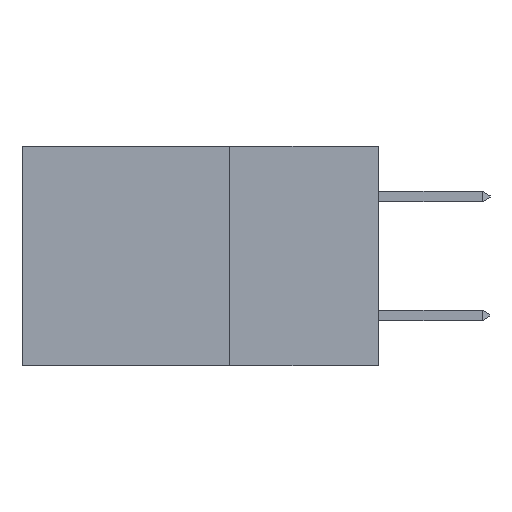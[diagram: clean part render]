
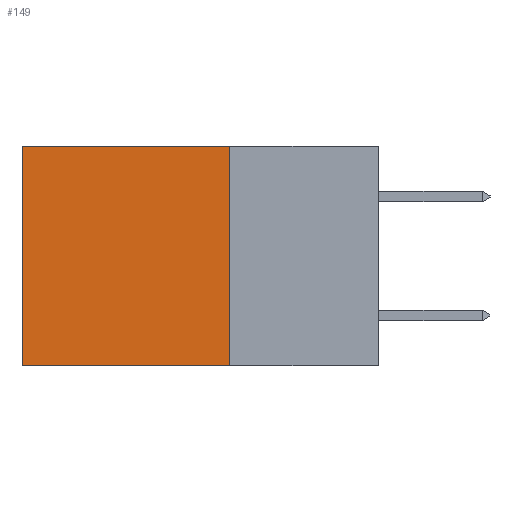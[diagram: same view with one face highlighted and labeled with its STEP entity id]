
A CAD part, left-side view. The second image highlights one B-rep face of the part: STEP entity #149.
In plain terms, the highlighted planar face has unit normal (-1, 0, 0).
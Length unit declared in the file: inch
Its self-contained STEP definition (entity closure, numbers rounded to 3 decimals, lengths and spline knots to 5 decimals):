
#149 = ADVANCED_FACE ( 'NONE', ( #1128 ), #3359, .F. ) ;
#1128 = FACE_OUTER_BOUND ( 'NONE', #11499, .T. ) ;
#1230 = CARTESIAN_POINT ( 'NONE',  ( 0.2615, 0.25, -0.37 ) ) ;
#1294 = DIRECTION ( 'NONE',  ( 0., 0., -1. ) ) ;
#1419 = DIRECTION ( 'NONE',  ( 0., 1., 0. ) ) ;
#2017 = CARTESIAN_POINT ( 'NONE',  ( 0.2615, 0.25, 0. ) ) ;
#2032 = LINE ( 'NONE', #10376, #15685 ) ;
#3327 = DIRECTION ( 'NONE',  ( 1., 0., 0. ) ) ;
#3359 = PLANE ( 'NONE',  #15931 ) ;
#3713 = ORIENTED_EDGE ( 'NONE', *, *, #17989, .T. ) ;
#4237 = VERTEX_POINT ( 'NONE', #5368 ) ;
#4998 = ORIENTED_EDGE ( 'NONE', *, *, #20909, .F. ) ;
#5368 = CARTESIAN_POINT ( 'NONE',  ( 0.2615, 0.6, -0.37 ) ) ;
#7786 = VECTOR ( 'NONE', #13307, 39.37008 ) ;
#8074 = DIRECTION ( 'NONE',  ( 0., 1., 0. ) ) ;
#8350 = DIRECTION ( 'NONE',  ( 0., 0., -1. ) ) ;
#10376 = CARTESIAN_POINT ( 'NONE',  ( 0.2615, 0.25, 0. ) ) ;
#11499 = EDGE_LOOP ( 'NONE', ( #3713, #20051, #4998, #11564 ) ) ;
#11564 = ORIENTED_EDGE ( 'NONE', *, *, #21011, .T. ) ;
#12499 = LINE ( 'NONE', #18508, #7786 ) ;
#13210 = VECTOR ( 'NONE', #8350, 39.37008 ) ;
#13307 = DIRECTION ( 'NONE',  ( 0., 0., -1. ) ) ;
#13685 = VERTEX_POINT ( 'NONE', #19286 ) ;
#14141 = EDGE_CURVE ( 'NONE', #21661, #4237, #21047, .T. ) ;
#15685 = VECTOR ( 'NONE', #1419, 39.37008 ) ;
#15931 = AXIS2_PLACEMENT_3D ( 'NONE', #20345, #3327, #1294 ) ;
#17144 = CARTESIAN_POINT ( 'NONE',  ( 0.2615, 0.25, -0.37 ) ) ;
#17446 = VECTOR ( 'NONE', #8074, 39.37008 ) ;
#17989 = EDGE_CURVE ( 'NONE', #13685, #4237, #12499, .T. ) ;
#18508 = CARTESIAN_POINT ( 'NONE',  ( 0.2615, 0.6, -0.37 ) ) ;
#18630 = CARTESIAN_POINT ( 'NONE',  ( 0.2615, 0.25, -0.37 ) ) ;
#19286 = CARTESIAN_POINT ( 'NONE',  ( 0.2615, 0.6, 0. ) ) ;
#20051 = ORIENTED_EDGE ( 'NONE', *, *, #14141, .F. ) ;
#20345 = CARTESIAN_POINT ( 'NONE',  ( 0.2615, 0.25, -0.37 ) ) ;
#20909 = EDGE_CURVE ( 'NONE', #22848, #21661, #21998, .T. ) ;
#21011 = EDGE_CURVE ( 'NONE', #22848, #13685, #2032, .T. ) ;
#21047 = LINE ( 'NONE', #18630, #17446 ) ;
#21661 = VERTEX_POINT ( 'NONE', #1230 ) ;
#21998 = LINE ( 'NONE', #17144, #13210 ) ;
#22848 = VERTEX_POINT ( 'NONE', #2017 ) ;
